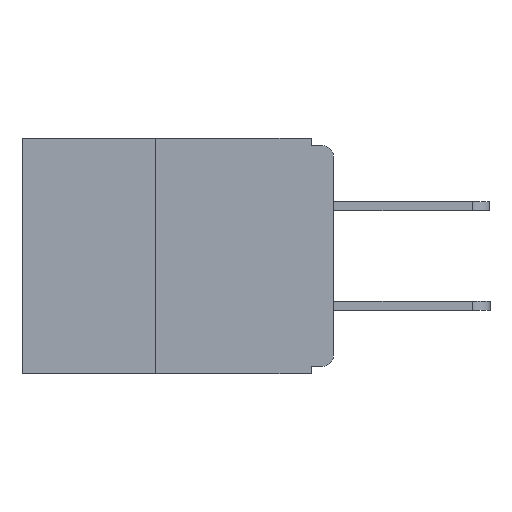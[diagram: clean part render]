
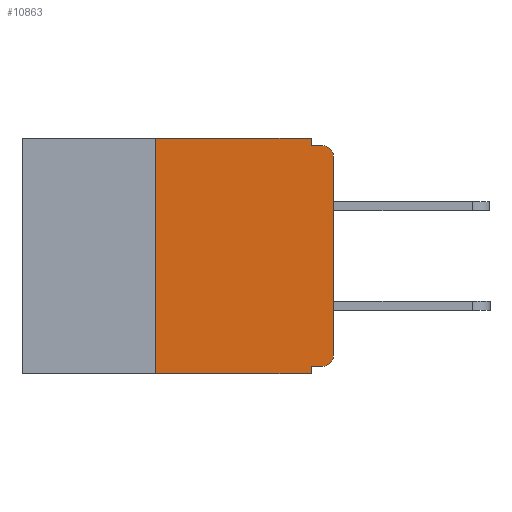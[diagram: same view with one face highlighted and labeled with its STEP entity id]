
A CAD part, left-side view. The second image highlights one B-rep face of the part: STEP entity #10863.
In plain terms, the highlighted planar face has unit normal (-1, 0, 0).
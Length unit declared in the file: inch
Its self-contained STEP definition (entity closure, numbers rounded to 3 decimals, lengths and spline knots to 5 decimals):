
#41 = VECTOR ( 'NONE', #8791, 39.37008 ) ;
#127 = CARTESIAN_POINT ( 'NONE',  ( 0., 0.25, -0.33 ) ) ;
#261 = CARTESIAN_POINT ( 'NONE',  ( 0., 0.015, -0.305 ) ) ;
#310 = LINE ( 'NONE', #12575, #4790 ) ;
#1037 = CARTESIAN_POINT ( 'NONE',  ( 0., 0., -0.305 ) ) ;
#1558 = ORIENTED_EDGE ( 'NONE', *, *, #10716, .F. ) ;
#1585 = EDGE_CURVE ( 'NONE', #4922, #10835, #12402, .T. ) ;
#1787 = DIRECTION ( 'NONE',  ( 0., 0., -1. ) ) ;
#2178 = EDGE_CURVE ( 'NONE', #14654, #4922, #15922, .T. ) ;
#2257 = DIRECTION ( 'NONE',  ( 0., 0., 1. ) ) ;
#2465 = CARTESIAN_POINT ( 'NONE',  ( 0., 0.25, -0.33 ) ) ;
#2503 = AXIS2_PLACEMENT_3D ( 'NONE', #12002, #7724, #17590 ) ;
#2630 = VECTOR ( 'NONE', #2257, 39.37008 ) ;
#2697 = ORIENTED_EDGE ( 'NONE', *, *, #2178, .T. ) ;
#2749 = VECTOR ( 'NONE', #11792, 39.37008 ) ;
#2923 = DIRECTION ( 'NONE',  ( 0., 1., 0. ) ) ;
#2953 = CARTESIAN_POINT ( 'NONE',  ( 0., 0., -0.32 ) ) ;
#3199 = ORIENTED_EDGE ( 'NONE', *, *, #6573, .F. ) ;
#3213 = LINE ( 'NONE', #13071, #7150 ) ;
#4020 = LINE ( 'NONE', #14496, #41 ) ;
#4313 = DIRECTION ( 'NONE',  ( 0., -1., 0. ) ) ;
#4431 = VECTOR ( 'NONE', #13226, 39.37008 ) ;
#4497 = CARTESIAN_POINT ( 'NONE',  ( 0., 0.437, -0.33 ) ) ;
#4790 = VECTOR ( 'NONE', #12633, 39.37008 ) ;
#4922 = VERTEX_POINT ( 'NONE', #17200 ) ;
#5192 = FACE_OUTER_BOUND ( 'NONE', #17432, .T. ) ;
#5351 = VERTEX_POINT ( 'NONE', #13408 ) ;
#5369 = VERTEX_POINT ( 'NONE', #12965 ) ;
#5433 = EDGE_CURVE ( 'NONE', #5351, #12206, #310, .T. ) ;
#6236 = ORIENTED_EDGE ( 'NONE', *, *, #5433, .F. ) ;
#6277 = PLANE ( 'NONE',  #2503 ) ;
#6415 = CARTESIAN_POINT ( 'NONE',  ( 0., 0.031, -0.33 ) ) ;
#6573 = EDGE_CURVE ( 'NONE', #7001, #5351, #15524, .T. ) ;
#6614 = LINE ( 'NONE', #2465, #2630 ) ;
#7001 = VERTEX_POINT ( 'NONE', #11870 ) ;
#7150 = VECTOR ( 'NONE', #14487, 39.37008 ) ;
#7724 = DIRECTION ( 'NONE',  ( 1., 0., 0. ) ) ;
#7741 = CARTESIAN_POINT ( 'NONE',  ( 0., 0.031, -0.01 ) ) ;
#7947 = VECTOR ( 'NONE', #2923, 39.37008 ) ;
#8382 = EDGE_CURVE ( 'NONE', #13729, #12206, #16888, .T. ) ;
#8487 = ORIENTED_EDGE ( 'NONE', *, *, #14255, .F. ) ;
#8745 = AXIS2_PLACEMENT_3D ( 'NONE', #261, #10586, #1787 ) ;
#8791 = DIRECTION ( 'NONE',  ( 0., -1., 0. ) ) ;
#10296 = EDGE_CURVE ( 'NONE', #13729, #5369, #6614, .T. ) ;
#10586 = DIRECTION ( 'NONE',  ( -1., 0., 0. ) ) ;
#10716 = EDGE_CURVE ( 'NONE', #5369, #10843, #4020, .T. ) ;
#10742 = ORIENTED_EDGE ( 'NONE', *, *, #10296, .F. ) ;
#10835 = VERTEX_POINT ( 'NONE', #13330 ) ;
#10843 = VERTEX_POINT ( 'NONE', #16146 ) ;
#10863 = ADVANCED_FACE ( 'NONE', ( #5192 ), #6277, .F. ) ;
#10884 = AXIS2_PLACEMENT_3D ( 'NONE', #11303, #15192, #17505 ) ;
#10961 = ORIENTED_EDGE ( 'NONE', *, *, #15542, .T. ) ;
#11303 = CARTESIAN_POINT ( 'NONE',  ( 0., 0.015, -0.025 ) ) ;
#11382 = ORIENTED_EDGE ( 'NONE', *, *, #1585, .T. ) ;
#11618 = ORIENTED_EDGE ( 'NONE', *, *, #8382, .T. ) ;
#11792 = DIRECTION ( 'NONE',  ( 0., 0., -1. ) ) ;
#11870 = CARTESIAN_POINT ( 'NONE',  ( 0., 0.015, -0.32 ) ) ;
#12002 = CARTESIAN_POINT ( 'NONE',  ( 0., 0.437, 0. ) ) ;
#12206 = VERTEX_POINT ( 'NONE', #6415 ) ;
#12402 = CIRCLE ( 'NONE', #10884, 0.015 ) ;
#12451 = CIRCLE ( 'NONE', #8745, 0.015 ) ;
#12575 = CARTESIAN_POINT ( 'NONE',  ( 0., 0.031, -0.33 ) ) ;
#12633 = DIRECTION ( 'NONE',  ( 0., 0., -1. ) ) ;
#12965 = CARTESIAN_POINT ( 'NONE',  ( 0., 0.25, 0. ) ) ;
#13071 = CARTESIAN_POINT ( 'NONE',  ( 0., 0., -0.01 ) ) ;
#13192 = EDGE_CURVE ( 'NONE', #10843, #15583, #17964, .T. ) ;
#13218 = VECTOR ( 'NONE', #4313, 39.37008 ) ;
#13226 = DIRECTION ( 'NONE',  ( 0., 0., 1. ) ) ;
#13330 = CARTESIAN_POINT ( 'NONE',  ( 0., 0.015, -0.01 ) ) ;
#13408 = CARTESIAN_POINT ( 'NONE',  ( 0., 0.031, -0.32 ) ) ;
#13535 = CARTESIAN_POINT ( 'NONE',  ( 0., 0., 0. ) ) ;
#13729 = VERTEX_POINT ( 'NONE', #127 ) ;
#14255 = EDGE_CURVE ( 'NONE', #15583, #10835, #3213, .T. ) ;
#14487 = DIRECTION ( 'NONE',  ( 0., -1., 0. ) ) ;
#14496 = CARTESIAN_POINT ( 'NONE',  ( 0., 0.437, 0. ) ) ;
#14654 = VERTEX_POINT ( 'NONE', #1037 ) ;
#15192 = DIRECTION ( 'NONE',  ( -1., 0., 0. ) ) ;
#15524 = LINE ( 'NONE', #2953, #7947 ) ;
#15542 = EDGE_CURVE ( 'NONE', #7001, #14654, #12451, .T. ) ;
#15583 = VERTEX_POINT ( 'NONE', #7741 ) ;
#15922 = LINE ( 'NONE', #13535, #4431 ) ;
#16146 = CARTESIAN_POINT ( 'NONE',  ( 0., 0.031, 0. ) ) ;
#16462 = ORIENTED_EDGE ( 'NONE', *, *, #13192, .F. ) ;
#16888 = LINE ( 'NONE', #4497, #13218 ) ;
#17200 = CARTESIAN_POINT ( 'NONE',  ( 0., 0., -0.025 ) ) ;
#17349 = CARTESIAN_POINT ( 'NONE',  ( 0., 0.031, 0. ) ) ;
#17432 = EDGE_LOOP ( 'NONE', ( #2697, #11382, #8487, #16462, #1558, #10742, #11618, #6236, #3199, #10961 ) ) ;
#17505 = DIRECTION ( 'NONE',  ( 0., 0., -1. ) ) ;
#17590 = DIRECTION ( 'NONE',  ( 0., 0., -1. ) ) ;
#17964 = LINE ( 'NONE', #17349, #2749 ) ;
